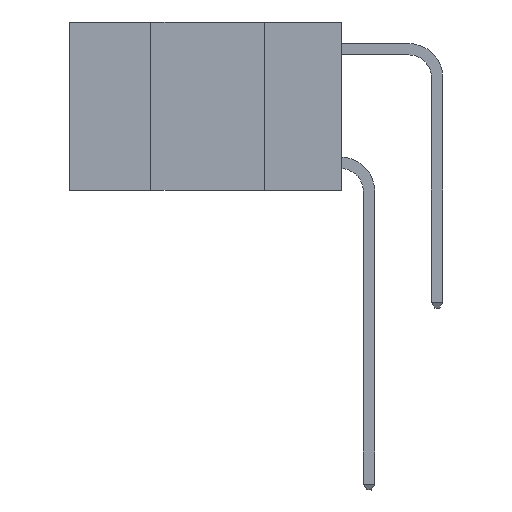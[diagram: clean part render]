
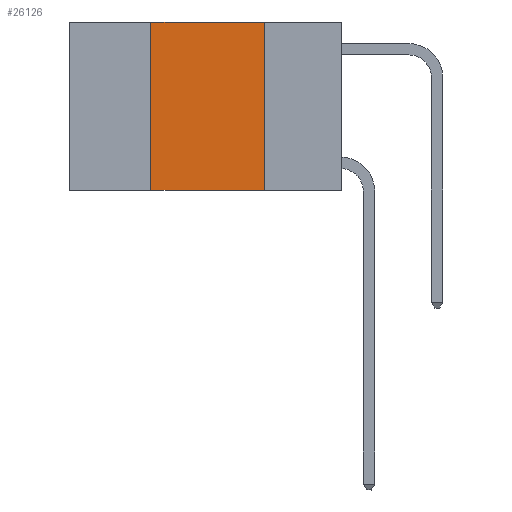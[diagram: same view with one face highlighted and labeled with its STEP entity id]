
A CAD part, left-side view. The second image highlights one B-rep face of the part: STEP entity #26126.
In plain terms, the highlighted planar face has unit normal (-1, 0, 0).
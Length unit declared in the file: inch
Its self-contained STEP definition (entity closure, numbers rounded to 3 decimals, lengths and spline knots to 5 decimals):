
#942 = VECTOR ( 'NONE', #10571, 39.37008 ) ;
#1546 = EDGE_CURVE ( 'NONE', #10686, #11832, #13183, .T. ) ;
#1746 = CARTESIAN_POINT ( 'NONE',  ( 0., 0.6, 0. ) ) ;
#3038 = DIRECTION ( 'NONE',  ( 0., -1., 0. ) ) ;
#6742 = EDGE_CURVE ( 'NONE', #12063, #10686, #17102, .T. ) ;
#7171 = CARTESIAN_POINT ( 'NONE',  ( 0., 0.17, -0.37 ) ) ;
#8081 = DIRECTION ( 'NONE',  ( 1., 0., 0. ) ) ;
#8211 = FACE_OUTER_BOUND ( 'NONE', #19801, .T. ) ;
#8954 = LINE ( 'NONE', #23464, #15731 ) ;
#10145 = DIRECTION ( 'NONE',  ( 0., 0., -1. ) ) ;
#10571 = DIRECTION ( 'NONE',  ( 0., -1., 0. ) ) ;
#10686 = VERTEX_POINT ( 'NONE', #14399 ) ;
#11224 = CARTESIAN_POINT ( 'NONE',  ( 0., 0.17, 0. ) ) ;
#11675 = EDGE_CURVE ( 'NONE', #11832, #25758, #19445, .T. ) ;
#11832 = VERTEX_POINT ( 'NONE', #11224 ) ;
#12063 = VERTEX_POINT ( 'NONE', #12420 ) ;
#12420 = CARTESIAN_POINT ( 'NONE',  ( 0., 0.42, -0.37 ) ) ;
#12892 = PLANE ( 'NONE',  #17188 ) ;
#12940 = VECTOR ( 'NONE', #23979, 39.37008 ) ;
#13183 = LINE ( 'NONE', #25481, #942 ) ;
#14399 = CARTESIAN_POINT ( 'NONE',  ( 0., 0.42, 0. ) ) ;
#15022 = DIRECTION ( 'NONE',  ( 0., 0., 1. ) ) ;
#15270 = CARTESIAN_POINT ( 'NONE',  ( 0., 0.17, 0. ) ) ;
#15731 = VECTOR ( 'NONE', #3038, 39.37008 ) ;
#15817 = VECTOR ( 'NONE', #15022, 39.37008 ) ;
#17102 = LINE ( 'NONE', #25504, #15817 ) ;
#17188 = AXIS2_PLACEMENT_3D ( 'NONE', #1746, #8081, #10145 ) ;
#18176 = ORIENTED_EDGE ( 'NONE', *, *, #1546, .F. ) ;
#19259 = EDGE_CURVE ( 'NONE', #12063, #25758, #8954, .T. ) ;
#19332 = ORIENTED_EDGE ( 'NONE', *, *, #11675, .F. ) ;
#19445 = LINE ( 'NONE', #15270, #12940 ) ;
#19801 = EDGE_LOOP ( 'NONE', ( #19332, #18176, #20673, #25318 ) ) ;
#20673 = ORIENTED_EDGE ( 'NONE', *, *, #6742, .F. ) ;
#23464 = CARTESIAN_POINT ( 'NONE',  ( 0., 0.6, -0.37 ) ) ;
#23979 = DIRECTION ( 'NONE',  ( 0., 0., -1. ) ) ;
#25318 = ORIENTED_EDGE ( 'NONE', *, *, #19259, .T. ) ;
#25481 = CARTESIAN_POINT ( 'NONE',  ( 0., 0.6, 0. ) ) ;
#25504 = CARTESIAN_POINT ( 'NONE',  ( 0., 0.42, 0. ) ) ;
#25758 = VERTEX_POINT ( 'NONE', #7171 ) ;
#26126 = ADVANCED_FACE ( 'NONE', ( #8211 ), #12892, .F. ) ;
